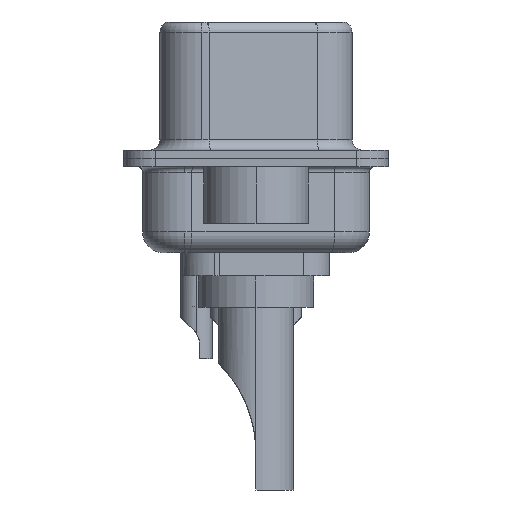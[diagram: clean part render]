
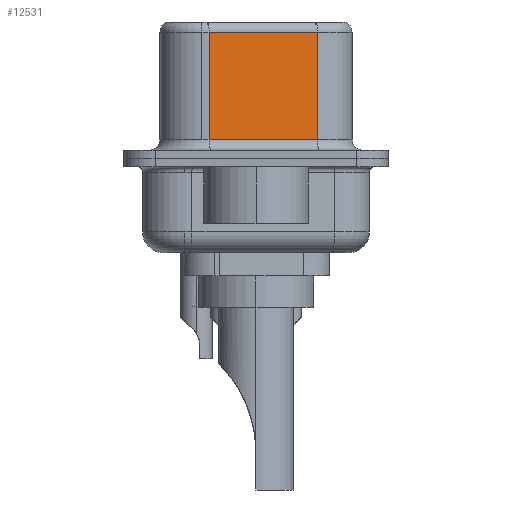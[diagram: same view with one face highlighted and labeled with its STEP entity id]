
A CAD part, left-side view. The second image highlights one B-rep face of the part: STEP entity #12531.
In plain terms, the highlighted planar face has unit normal (-0.985, -0.174, 0).
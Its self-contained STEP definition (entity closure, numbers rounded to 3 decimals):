
#1027 = VERTEX_POINT ( 'NONE', #13173 ) ;
#1040 = VERTEX_POINT ( 'NONE', #1816 ) ;
#1334 = LINE ( 'NONE', #18506, #9775 ) ;
#1692 = ORIENTED_EDGE ( 'NONE', *, *, #14322, .T. ) ;
#1816 = CARTESIAN_POINT ( 'NONE',  ( 3.67, 2.233, 6.02 ) ) ;
#1897 = VERTEX_POINT ( 'NONE', #6253 ) ;
#2684 = VECTOR ( 'NONE', #17227, 1000. ) ;
#2761 = ORIENTED_EDGE ( 'NONE', *, *, #19701, .T. ) ;
#2783 = ORIENTED_EDGE ( 'NONE', *, *, #15292, .T. ) ;
#4024 = ORIENTED_EDGE ( 'NONE', *, *, #15676, .F. ) ;
#5140 = AXIS2_PLACEMENT_3D ( 'NONE', #12988, #17813, #8230 ) ;
#6253 = CARTESIAN_POINT ( 'NONE',  ( 3.67, 2.233, 0.9 ) ) ;
#6822 = FACE_OUTER_BOUND ( 'NONE', #17385, .T. ) ;
#8230 = DIRECTION ( 'NONE',  ( -0.174, 0.985, 0. ) ) ;
#9775 = VECTOR ( 'NONE', #18217, 1000. ) ;
#10366 = VECTOR ( 'NONE', #14399, 1000. ) ;
#11243 = CARTESIAN_POINT ( 'NONE',  ( 4.58, -2.927, 0.9 ) ) ;
#11409 = PLANE ( 'NONE',  #5140 ) ;
#11847 = LINE ( 'NONE', #17538, #10366 ) ;
#11854 = CARTESIAN_POINT ( 'NONE',  ( 4.58, -2.927, 0.9 ) ) ;
#12531 = ADVANCED_FACE ( 'NONE', ( #6822 ), #11409, .F. ) ;
#12988 = CARTESIAN_POINT ( 'NONE',  ( 4.58, -2.927, 6.52 ) ) ;
#13173 = CARTESIAN_POINT ( 'NONE',  ( 4.58, -2.927, 6.02 ) ) ;
#13775 = LINE ( 'NONE', #14020, #2684 ) ;
#14020 = CARTESIAN_POINT ( 'NONE',  ( 4.58, -2.927, 6.52 ) ) ;
#14322 = EDGE_CURVE ( 'NONE', #1040, #1897, #11847, .T. ) ;
#14399 = DIRECTION ( 'NONE',  ( 0., 0., -1. ) ) ;
#15292 = EDGE_CURVE ( 'NONE', #1897, #18290, #19824, .T. ) ;
#15531 = VECTOR ( 'NONE', #19210, 1000. ) ;
#15676 = EDGE_CURVE ( 'NONE', #1027, #18290, #13775, .T. ) ;
#17227 = DIRECTION ( 'NONE',  ( 0., 0., -1. ) ) ;
#17385 = EDGE_LOOP ( 'NONE', ( #4024, #2761, #1692, #2783 ) ) ;
#17538 = CARTESIAN_POINT ( 'NONE',  ( 3.67, 2.233, 6.52 ) ) ;
#17813 = DIRECTION ( 'NONE',  ( 0.985, 0.174, 0. ) ) ;
#18217 = DIRECTION ( 'NONE',  ( -0.174, 0.985, 0. ) ) ;
#18290 = VERTEX_POINT ( 'NONE', #11854 ) ;
#18506 = CARTESIAN_POINT ( 'NONE',  ( 4.58, -2.927, 6.02 ) ) ;
#19210 = DIRECTION ( 'NONE',  ( 0.174, -0.985, 0. ) ) ;
#19701 = EDGE_CURVE ( 'NONE', #1027, #1040, #1334, .T. ) ;
#19824 = LINE ( 'NONE', #11243, #15531 ) ;
